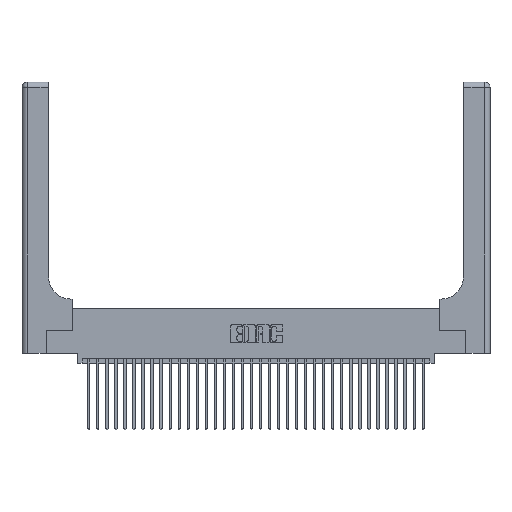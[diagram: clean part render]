
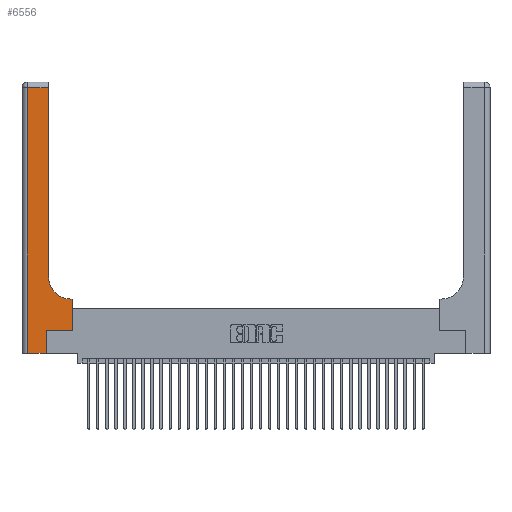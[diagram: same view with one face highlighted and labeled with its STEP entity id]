
A CAD part, top view. The second image highlights one B-rep face of the part: STEP entity #6556.
In plain terms, the highlighted planar face has unit normal (0, 0, 1).
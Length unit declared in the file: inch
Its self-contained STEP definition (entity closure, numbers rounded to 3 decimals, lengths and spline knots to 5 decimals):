
#311 = DIRECTION ( 'NONE',  ( -1., 0., 0. ) ) ;
#545 = DIRECTION ( 'NONE',  ( -1., 0., 0. ) ) ;
#556 = ORIENTED_EDGE ( 'NONE', *, *, #19722, .T. ) ;
#559 = VECTOR ( 'NONE', #18989, 39.37008 ) ;
#889 = DIRECTION ( 'NONE',  ( 1., 0., 0. ) ) ;
#2449 = CARTESIAN_POINT ( 'NONE',  ( 0.06, 0., 0.37 ) ) ;
#3856 = VERTEX_POINT ( 'NONE', #31115 ) ;
#4160 = VECTOR ( 'NONE', #16588, 39.37008 ) ;
#4253 = FACE_OUTER_BOUND ( 'NONE', #4698, .T. ) ;
#4537 = CARTESIAN_POINT ( 'NONE',  ( 0.5585, 0.25, 0.37 ) ) ;
#4698 = EDGE_LOOP ( 'NONE', ( #12668, #27314, #13554, #29034, #556, #30756, #9641, #32470, #11380 ) ) ;
#4886 = CARTESIAN_POINT ( 'NONE',  ( 0.2915, 0.6, 0.37 ) ) ;
#5635 = DIRECTION ( 'NONE',  ( 0., -1., 0. ) ) ;
#6316 = VECTOR ( 'NONE', #7311, 39.37008 ) ;
#6322 = VERTEX_POINT ( 'NONE', #26849 ) ;
#6556 = ADVANCED_FACE ( 'NONE', ( #4253 ), #33320, .F. ) ;
#6607 = EDGE_CURVE ( 'NONE', #30905, #26285, #9864, .T. ) ;
#6875 = DIRECTION ( 'NONE',  ( 1., 0., 0. ) ) ;
#7311 = DIRECTION ( 'NONE',  ( 0., 1., 0. ) ) ;
#8314 = VERTEX_POINT ( 'NONE', #14263 ) ;
#8648 = VERTEX_POINT ( 'NONE', #15816 ) ;
#8665 = CARTESIAN_POINT ( 'NONE',  ( 0., 2.94, 0.37 ) ) ;
#9527 = CARTESIAN_POINT ( 'NONE',  ( 0.269, 0.25, 0.37 ) ) ;
#9641 = ORIENTED_EDGE ( 'NONE', *, *, #27468, .T. ) ;
#9864 = LINE ( 'NONE', #8665, #30975 ) ;
#10018 = AXIS2_PLACEMENT_3D ( 'NONE', #19565, #16881, #311 ) ;
#10636 = LINE ( 'NONE', #30291, #4160 ) ;
#10767 = CARTESIAN_POINT ( 'NONE',  ( 0.06, 2.94, 0.37 ) ) ;
#11380 = ORIENTED_EDGE ( 'NONE', *, *, #18628, .T. ) ;
#11570 = CARTESIAN_POINT ( 'NONE',  ( 0.5415, 0.85, 0.37 ) ) ;
#11727 = EDGE_CURVE ( 'NONE', #17734, #18111, #28486, .T. ) ;
#12668 = ORIENTED_EDGE ( 'NONE', *, *, #29987, .T. ) ;
#13554 = ORIENTED_EDGE ( 'NONE', *, *, #14219, .T. ) ;
#13845 = VECTOR ( 'NONE', #889, 39.37008 ) ;
#14219 = EDGE_CURVE ( 'NONE', #26285, #17734, #22796, .T. ) ;
#14263 = CARTESIAN_POINT ( 'NONE',  ( 0.2915, 0.85, 0.37 ) ) ;
#14340 = DIRECTION ( 'NONE',  ( 1., 0., 0. ) ) ;
#15263 = LINE ( 'NONE', #16195, #559 ) ;
#15439 = VECTOR ( 'NONE', #5635, 39.37008 ) ;
#15816 = CARTESIAN_POINT ( 'NONE',  ( 0.5585, 0.6, 0.37 ) ) ;
#15914 = CIRCLE ( 'NONE', #33065, 0.25 ) ;
#16007 = DIRECTION ( 'NONE',  ( -1., 0., 0. ) ) ;
#16195 = CARTESIAN_POINT ( 'NONE',  ( 0.2915, 3., 0.37 ) ) ;
#16588 = DIRECTION ( 'NONE',  ( 0., 1., 0. ) ) ;
#16801 = LINE ( 'NONE', #9527, #22420 ) ;
#16881 = DIRECTION ( 'NONE',  ( 0., 0., -1. ) ) ;
#17734 = VERTEX_POINT ( 'NONE', #2449 ) ;
#18111 = VERTEX_POINT ( 'NONE', #25928 ) ;
#18202 = CARTESIAN_POINT ( 'NONE',  ( 0.2915, 2.94, 0.37 ) ) ;
#18628 = EDGE_CURVE ( 'NONE', #3856, #8314, #15914, .T. ) ;
#18989 = DIRECTION ( 'NONE',  ( 0., 1., 0. ) ) ;
#19440 = CARTESIAN_POINT ( 'NONE',  ( 0.06, 3., 0.37 ) ) ;
#19565 = CARTESIAN_POINT ( 'NONE',  ( 0., 3., 0.37 ) ) ;
#19722 = EDGE_CURVE ( 'NONE', #18111, #6322, #10636, .T. ) ;
#20274 = CARTESIAN_POINT ( 'NONE',  ( 0., 0., 0.37 ) ) ;
#21040 = LINE ( 'NONE', #4537, #6316 ) ;
#22420 = VECTOR ( 'NONE', #6875, 39.37008 ) ;
#22553 = CARTESIAN_POINT ( 'NONE',  ( 0.5585, 0.25, 0.37 ) ) ;
#22796 = LINE ( 'NONE', #19440, #15439 ) ;
#25928 = CARTESIAN_POINT ( 'NONE',  ( 0.269, 0., 0.37 ) ) ;
#26285 = VERTEX_POINT ( 'NONE', #10767 ) ;
#26429 = VECTOR ( 'NONE', #16007, 39.37008 ) ;
#26849 = CARTESIAN_POINT ( 'NONE',  ( 0.269, 0.25, 0.37 ) ) ;
#27308 = LINE ( 'NONE', #4886, #26429 ) ;
#27314 = ORIENTED_EDGE ( 'NONE', *, *, #6607, .T. ) ;
#27468 = EDGE_CURVE ( 'NONE', #28931, #8648, #21040, .T. ) ;
#28486 = LINE ( 'NONE', #20274, #13845 ) ;
#28931 = VERTEX_POINT ( 'NONE', #22553 ) ;
#29034 = ORIENTED_EDGE ( 'NONE', *, *, #11727, .T. ) ;
#29987 = EDGE_CURVE ( 'NONE', #8314, #30905, #15263, .T. ) ;
#30291 = CARTESIAN_POINT ( 'NONE',  ( 0.269, 0., 0.37 ) ) ;
#30756 = ORIENTED_EDGE ( 'NONE', *, *, #33662, .T. ) ;
#30821 = DIRECTION ( 'NONE',  ( 0., 0., -1. ) ) ;
#30905 = VERTEX_POINT ( 'NONE', #18202 ) ;
#30975 = VECTOR ( 'NONE', #545, 39.37008 ) ;
#31048 = EDGE_CURVE ( 'NONE', #8648, #3856, #27308, .T. ) ;
#31115 = CARTESIAN_POINT ( 'NONE',  ( 0.5415, 0.6, 0.37 ) ) ;
#32470 = ORIENTED_EDGE ( 'NONE', *, *, #31048, .T. ) ;
#33065 = AXIS2_PLACEMENT_3D ( 'NONE', #11570, #30821, #14340 ) ;
#33320 = PLANE ( 'NONE',  #10018 ) ;
#33662 = EDGE_CURVE ( 'NONE', #6322, #28931, #16801, .T. ) ;
